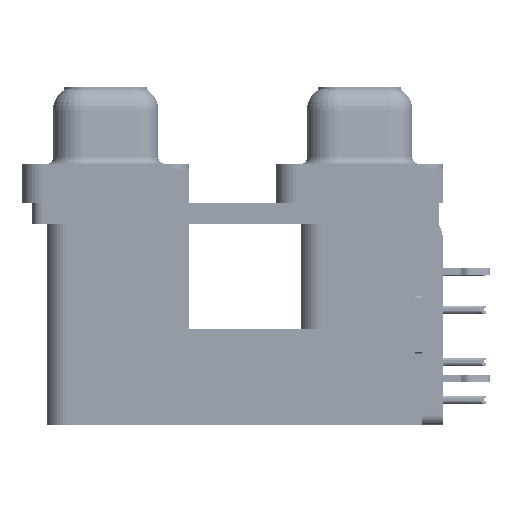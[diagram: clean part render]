
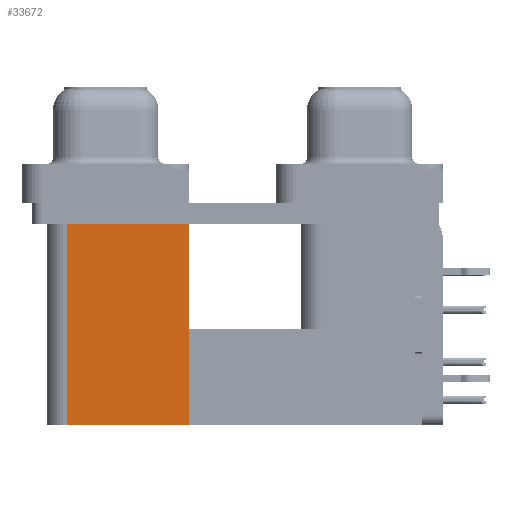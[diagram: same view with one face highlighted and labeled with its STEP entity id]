
A CAD part, left-side view. The second image highlights one B-rep face of the part: STEP entity #33672.
In plain terms, the highlighted planar face has unit normal (-1, 0, 0).
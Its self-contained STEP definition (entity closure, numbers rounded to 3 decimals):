
#3156 = FACE_OUTER_BOUND ( 'NONE', #41494, .T. ) ;
#3622 = ORIENTED_EDGE ( 'NONE', *, *, #18966, .T. ) ;
#6399 = LINE ( 'NONE', #54258, #34235 ) ;
#10137 = ORIENTED_EDGE ( 'NONE', *, *, #23546, .F. ) ;
#10433 = VERTEX_POINT ( 'NONE', #55764 ) ;
#10560 = DIRECTION ( 'NONE',  ( 0., 0., 1. ) ) ;
#10739 = DIRECTION ( 'NONE',  ( 0., 1., 0. ) ) ;
#11996 = VERTEX_POINT ( 'NONE', #61825 ) ;
#13472 = LINE ( 'NONE', #45774, #22485 ) ;
#14218 = DIRECTION ( 'NONE',  ( 1., 0., 0. ) ) ;
#15232 = LINE ( 'NONE', #30492, #56800 ) ;
#15996 = CARTESIAN_POINT ( 'NONE',  ( 3.7, 21.975, -19.2 ) ) ;
#18966 = EDGE_CURVE ( 'NONE', #10433, #11996, #29440, .T. ) ;
#22485 = VECTOR ( 'NONE', #50565, 1000. ) ;
#23546 = EDGE_CURVE ( 'NONE', #10433, #30083, #13472, .T. ) ;
#29440 = LINE ( 'NONE', #52757, #49297 ) ;
#30083 = VERTEX_POINT ( 'NONE', #15996 ) ;
#30492 = CARTESIAN_POINT ( 'NONE',  ( 3.7, 12.775, -2.5 ) ) ;
#31612 = ORIENTED_EDGE ( 'NONE', *, *, #60611, .F. ) ;
#33672 = ADVANCED_FACE ( 'NONE', ( #3156 ), #46209, .F. ) ;
#34235 = VECTOR ( 'NONE', #10560, 1000. ) ;
#34271 = VERTEX_POINT ( 'NONE', #59186 ) ;
#35420 = AXIS2_PLACEMENT_3D ( 'NONE', #41425, #14218, #60903 ) ;
#38853 = EDGE_CURVE ( 'NONE', #11996, #34271, #15232, .T. ) ;
#41425 = CARTESIAN_POINT ( 'NONE',  ( 3.7, 12.775, -19.2 ) ) ;
#41494 = EDGE_LOOP ( 'NONE', ( #60819, #31612, #10137, #3622 ) ) ;
#43184 = DIRECTION ( 'NONE',  ( 0., 0., 1. ) ) ;
#45774 = CARTESIAN_POINT ( 'NONE',  ( 3.7, 12.775, -19.2 ) ) ;
#46209 = PLANE ( 'NONE',  #35420 ) ;
#49297 = VECTOR ( 'NONE', #43184, 1000. ) ;
#50565 = DIRECTION ( 'NONE',  ( 0., 1., 0. ) ) ;
#52757 = CARTESIAN_POINT ( 'NONE',  ( 3.7, 12.775, -19.2 ) ) ;
#54258 = CARTESIAN_POINT ( 'NONE',  ( 3.7, 21.975, -19.2 ) ) ;
#55764 = CARTESIAN_POINT ( 'NONE',  ( 3.7, 12.775, -19.2 ) ) ;
#56800 = VECTOR ( 'NONE', #10739, 1000. ) ;
#59186 = CARTESIAN_POINT ( 'NONE',  ( 3.7, 21.975, -2.5 ) ) ;
#60611 = EDGE_CURVE ( 'NONE', #30083, #34271, #6399, .T. ) ;
#60819 = ORIENTED_EDGE ( 'NONE', *, *, #38853, .T. ) ;
#60903 = DIRECTION ( 'NONE',  ( 0., 1., 0. ) ) ;
#61825 = CARTESIAN_POINT ( 'NONE',  ( 3.7, 12.775, -2.5 ) ) ;
